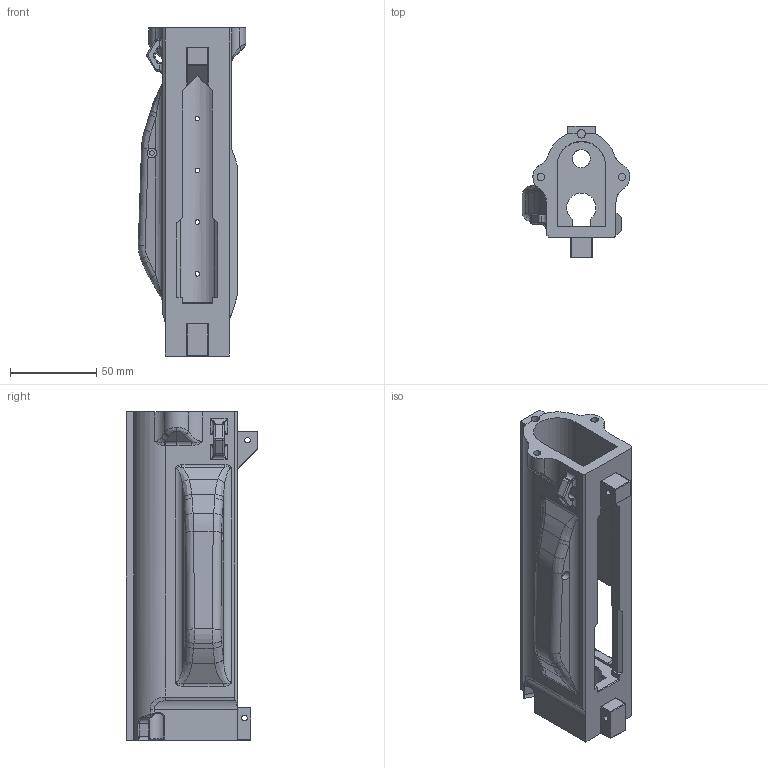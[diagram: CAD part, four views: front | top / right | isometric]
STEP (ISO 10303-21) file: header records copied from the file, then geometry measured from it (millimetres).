
FILE_DESCRIPTION(/* description */ (''),/* implementation_level */ '2;1');
FILE_NAME(/* name */ 'Upper Receiver.step',/* time_stamp */ '2022-05-11T21:22:43-06:00',/* author */ (''),/* organization */ (''),/* preprocessor_version */ 'ST-DEVELOPER v18.1',/* originating_system */ 'Autodesk Translation Framework v10.10.0.1391',/* authorisation */ '');
FILE_SCHEMA (('AUTOMOTIVE_DESIGN { 1 0 10303 214 3 1 1 }'));
Length unit declared in the file: millimetre
Products named in the file (1): Upper Receiver
Bounding box: 62.37 x 76.47 x 190.38 mm (x, y, z)
Volume: 206160.2 mm3; surface area: 72255.1 mm2
Topology: 1 solids, 2 shells, 345 faces, 853 edges, 510 vertices
Faces by surface type: cylinder 124, plane 118, bspline 73, torus 15, sphere 8, cone 7
Full cylindrical faces by diameter (mm): 2.65 x8, 2.7 x4, 3 x7, 3.2 x1, 3.3 x1, 4.35 x2, 4.5 x3, 4.9 x1, 5.65 x1, 10.5 x1, 28.3 x1
Entity records: 12389 total; most frequent: CARTESIAN_POINT 4476, ORIENTED_EDGE 1668, DIRECTION 1575, EDGE_CURVE 834, AXIS2_PLACEMENT_3D 589, VERTEX_POINT 510, LINE 397, VECTOR 397
